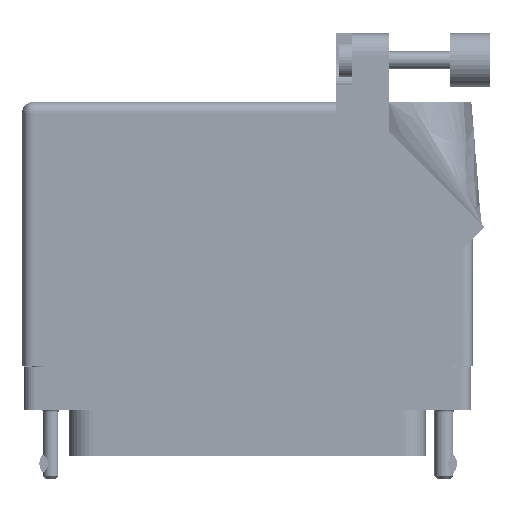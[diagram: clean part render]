
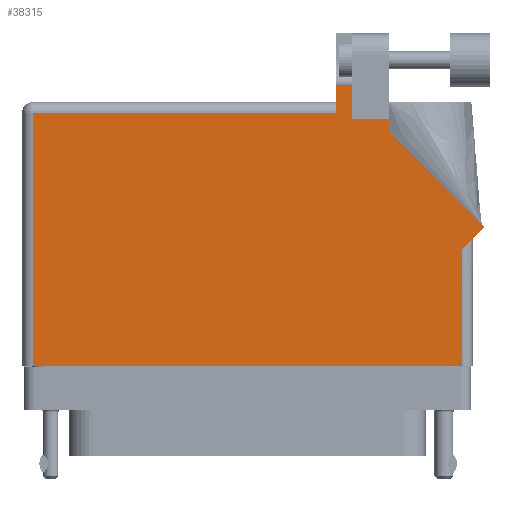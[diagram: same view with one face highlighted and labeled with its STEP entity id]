
A CAD part, front view. The second image highlights one B-rep face of the part: STEP entity #38315.
In plain terms, the highlighted face is planar.
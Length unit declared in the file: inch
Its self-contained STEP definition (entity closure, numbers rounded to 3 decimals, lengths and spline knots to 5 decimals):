
#28 = CARTESIAN_POINT ( 'NONE',  ( 0.607, 1.5315, 0.455 ) ) ;
#809 = EDGE_CURVE ( 'NONE', #35195, #16317, #20052, .T. ) ;
#962 = EDGE_CURVE ( 'NONE', #43939, #51893, #52578, .T. ) ;
#982 = VERTEX_POINT ( 'NONE', #55798 ) ;
#1414 = ORIENTED_EDGE ( 'NONE', *, *, #809, .T. ) ;
#2368 = DIRECTION ( 'NONE',  ( 0.707, 0.707, 0. ) ) ;
#2416 = CARTESIAN_POINT ( 'NONE',  ( -1.244, -0.1, 0.455 ) ) ;
#2656 = CARTESIAN_POINT ( 'NONE',  ( -1.306, 1.43, 0.455 ) ) ;
#4104 = DIRECTION ( 'NONE',  ( 0., 1., 0. ) ) ;
#4355 = CARTESIAN_POINT ( 'NONE',  ( 0.82, 1.26442, 0.455 ) ) ;
#4472 = EDGE_CURVE ( 'NONE', #26773, #24233, #33369, .T. ) ;
#5235 = LINE ( 'NONE', #2416, #28942 ) ;
#6593 = DIRECTION ( 'NONE',  ( 0., -1., 0. ) ) ;
#7560 = DIRECTION ( 'NONE',  ( 0., 1., 0. ) ) ;
#7784 = DIRECTION ( 'NONE',  ( -1., 0., 0. ) ) ;
#8108 = VECTOR ( 'NONE', #7560, 39.37008 ) ;
#8740 = EDGE_CURVE ( 'NONE', #24233, #38931, #5235, .T. ) ;
#9058 = ORIENTED_EDGE ( 'NONE', *, *, #36039, .T. ) ;
#9239 = LINE ( 'NONE', #50813, #23362 ) ;
#9363 = ORIENTED_EDGE ( 'NONE', *, *, #40090, .T. ) ;
#9475 = EDGE_CURVE ( 'NONE', #52237, #35195, #32200, .T. ) ;
#9541 = ORIENTED_EDGE ( 'NONE', *, *, #9475, .T. ) ;
#9562 = CARTESIAN_POINT ( 'NONE',  ( -1.244, -0.1, 0.455 ) ) ;
#10186 = AXIS2_PLACEMENT_3D ( 'NONE', #2656, #40656, #45452 ) ;
#11406 = DIRECTION ( 'NONE',  ( -1., 0., 0. ) ) ;
#13225 = LINE ( 'NONE', #14791, #13919 ) ;
#13919 = VECTOR ( 'NONE', #24748, 39.37008 ) ;
#14791 = CARTESIAN_POINT ( 'NONE',  ( 0.82, 1.33, 0.455 ) ) ;
#16317 = VERTEX_POINT ( 'NONE', #16657 ) ;
#16527 = VECTOR ( 'NONE', #2368, 39.37008 ) ;
#16657 = CARTESIAN_POINT ( 'NONE',  ( 0.82, 1.33, 0.455 ) ) ;
#17048 = CARTESIAN_POINT ( 'NONE',  ( 1.244, 0.575, 0.455 ) ) ;
#17642 = EDGE_CURVE ( 'NONE', #53224, #52237, #29152, .T. ) ;
#18191 = VECTOR ( 'NONE', #41821, 39.37008 ) ;
#19953 = CARTESIAN_POINT ( 'NONE',  ( -1.244, 1.368, 0.455 ) ) ;
#19993 = EDGE_LOOP ( 'NONE', ( #50004, #29438, #9363, #32902, #53733, #48695, #9058, #42877, #9541, #1414, #23032 ) ) ;
#20052 = LINE ( 'NONE', #54372, #28369 ) ;
#22296 = CARTESIAN_POINT ( 'NONE',  ( 1.306, 0.637, 0.455 ) ) ;
#23032 = ORIENTED_EDGE ( 'NONE', *, *, #53874, .T. ) ;
#23362 = VECTOR ( 'NONE', #41068, 39.37008 ) ;
#24233 = VERTEX_POINT ( 'NONE', #19953 ) ;
#24748 = DIRECTION ( 'NONE',  ( -1., 0., 0. ) ) ;
#26517 = CARTESIAN_POINT ( 'NONE',  ( 1.37671, 0.70771, 0.455 ) ) ;
#26773 = VERTEX_POINT ( 'NONE', #42861 ) ;
#28369 = VECTOR ( 'NONE', #30686, 39.37008 ) ;
#28942 = VECTOR ( 'NONE', #6593, 39.37008 ) ;
#29152 = LINE ( 'NONE', #22296, #16527 ) ;
#29438 = ORIENTED_EDGE ( 'NONE', *, *, #51074, .T. ) ;
#30686 = DIRECTION ( 'NONE',  ( 0., 1., 0. ) ) ;
#31986 = CARTESIAN_POINT ( 'NONE',  ( 0.513, 1.5315, 0.455 ) ) ;
#32200 = LINE ( 'NONE', #58668, #59731 ) ;
#32902 = ORIENTED_EDGE ( 'NONE', *, *, #4472, .T. ) ;
#33369 = LINE ( 'NONE', #54160, #54201 ) ;
#34099 = LINE ( 'NONE', #54695, #8108 ) ;
#34976 = LINE ( 'NONE', #46225, #49128 ) ;
#35195 = VERTEX_POINT ( 'NONE', #4355 ) ;
#36039 = EDGE_CURVE ( 'NONE', #982, #53224, #34099, .T. ) ;
#37124 = CARTESIAN_POINT ( 'NONE',  ( 0.607, 1.33, 0.455 ) ) ;
#37663 = VECTOR ( 'NONE', #4104, 39.37008 ) ;
#38315 = ADVANCED_FACE ( 'NONE', ( #61425 ), #49798, .F. ) ;
#38931 = VERTEX_POINT ( 'NONE', #9562 ) ;
#40090 = EDGE_CURVE ( 'NONE', #60425, #26773, #9239, .T. ) ;
#40656 = DIRECTION ( 'NONE',  ( 0., 0., -1. ) ) ;
#41068 = DIRECTION ( 'NONE',  ( 0., -1., 0. ) ) ;
#41821 = DIRECTION ( 'NONE',  ( 1., 0., 0. ) ) ;
#42861 = CARTESIAN_POINT ( 'NONE',  ( 0.513, 1.368, 0.455 ) ) ;
#42877 = ORIENTED_EDGE ( 'NONE', *, *, #17642, .T. ) ;
#43939 = VERTEX_POINT ( 'NONE', #44898 ) ;
#44898 = CARTESIAN_POINT ( 'NONE',  ( 0.607, 1.33, 0.455 ) ) ;
#45452 = DIRECTION ( 'NONE',  ( -1., 0., 0. ) ) ;
#46225 = CARTESIAN_POINT ( 'NONE',  ( 0.93777, 1.5315, 0.455 ) ) ;
#48695 = ORIENTED_EDGE ( 'NONE', *, *, #61320, .T. ) ;
#49128 = VECTOR ( 'NONE', #7784, 39.37008 ) ;
#49798 = PLANE ( 'NONE',  #10186 ) ;
#50004 = ORIENTED_EDGE ( 'NONE', *, *, #962, .T. ) ;
#50813 = CARTESIAN_POINT ( 'NONE',  ( 0.513, 1.43, 0.455 ) ) ;
#51074 = EDGE_CURVE ( 'NONE', #51893, #60425, #34976, .T. ) ;
#51893 = VERTEX_POINT ( 'NONE', #28 ) ;
#52237 = VERTEX_POINT ( 'NONE', #26517 ) ;
#52578 = LINE ( 'NONE', #37124, #37663 ) ;
#53224 = VERTEX_POINT ( 'NONE', #17048 ) ;
#53733 = ORIENTED_EDGE ( 'NONE', *, *, #8740, .T. ) ;
#53874 = EDGE_CURVE ( 'NONE', #16317, #43939, #13225, .T. ) ;
#53911 = LINE ( 'NONE', #61125, #18191 ) ;
#54160 = CARTESIAN_POINT ( 'NONE',  ( -1.306, 1.368, 0.455 ) ) ;
#54201 = VECTOR ( 'NONE', #11406, 39.37008 ) ;
#54372 = CARTESIAN_POINT ( 'NONE',  ( 0.82, 1.26442, 0.455 ) ) ;
#54695 = CARTESIAN_POINT ( 'NONE',  ( 1.244, 0.637, 0.455 ) ) ;
#55798 = CARTESIAN_POINT ( 'NONE',  ( 1.244, -0.1, 0.455 ) ) ;
#58233 = DIRECTION ( 'NONE',  ( -0.707, 0.707, 0. ) ) ;
#58668 = CARTESIAN_POINT ( 'NONE',  ( 1.37671, 0.70771, 0.455 ) ) ;
#59731 = VECTOR ( 'NONE', #58233, 39.37008 ) ;
#60425 = VERTEX_POINT ( 'NONE', #31986 ) ;
#61125 = CARTESIAN_POINT ( 'NONE',  ( -1.306, -0.1, 0.455 ) ) ;
#61320 = EDGE_CURVE ( 'NONE', #38931, #982, #53911, .T. ) ;
#61425 = FACE_OUTER_BOUND ( 'NONE', #19993, .T. ) ;
